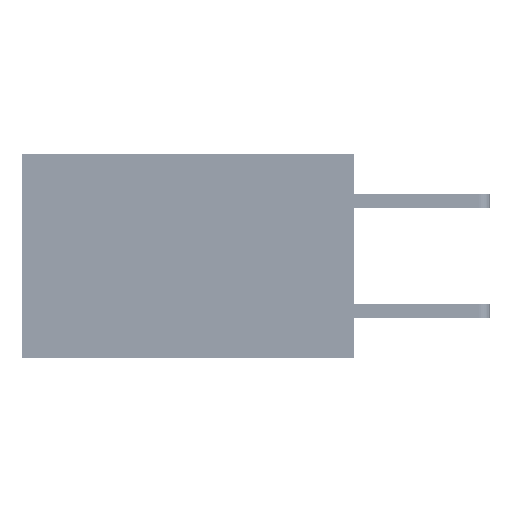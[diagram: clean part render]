
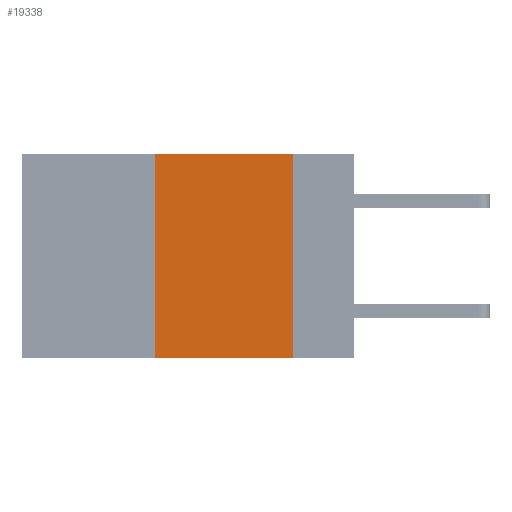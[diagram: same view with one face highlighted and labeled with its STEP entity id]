
A CAD part, left-side view. The second image highlights one B-rep face of the part: STEP entity #19338.
In plain terms, the highlighted planar face has unit normal (-1, 0, 0).
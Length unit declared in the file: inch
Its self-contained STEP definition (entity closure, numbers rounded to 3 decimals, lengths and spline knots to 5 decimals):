
#36 = CARTESIAN_POINT ( 'NONE',  ( 0., 0.11, 0. ) ) ;
#203 = DIRECTION ( 'NONE',  ( 0., -1., 0. ) ) ;
#1530 = VERTEX_POINT ( 'NONE', #18561 ) ;
#1953 = LINE ( 'NONE', #26231, #17473 ) ;
#5167 = ORIENTED_EDGE ( 'NONE', *, *, #29840, .F. ) ;
#6471 = VERTEX_POINT ( 'NONE', #21093 ) ;
#7067 = VECTOR ( 'NONE', #14658, 39.37008 ) ;
#13841 = VECTOR ( 'NONE', #46342, 39.37008 ) ;
#14285 = EDGE_CURVE ( 'NONE', #43423, #21439, #18416, .T. ) ;
#14658 = DIRECTION ( 'NONE',  ( 0., 0., -1. ) ) ;
#16258 = CARTESIAN_POINT ( 'NONE',  ( 0., 0.11, 0. ) ) ;
#16820 = PLANE ( 'NONE',  #38853 ) ;
#17473 = VECTOR ( 'NONE', #40788, 39.37008 ) ;
#18416 = LINE ( 'NONE', #36, #7067 ) ;
#18561 = CARTESIAN_POINT ( 'NONE',  ( 0., 0.36, -0.37 ) ) ;
#19338 = ADVANCED_FACE ( 'NONE', ( #24798 ), #16820, .F. ) ;
#19542 = CARTESIAN_POINT ( 'NONE',  ( 0., 0.11, -0.37 ) ) ;
#20822 = CARTESIAN_POINT ( 'NONE',  ( 0., 0.6, 0. ) ) ;
#21093 = CARTESIAN_POINT ( 'NONE',  ( 0., 0.36, 0. ) ) ;
#21439 = VERTEX_POINT ( 'NONE', #19542 ) ;
#24097 = VECTOR ( 'NONE', #203, 39.37008 ) ;
#24798 = FACE_OUTER_BOUND ( 'NONE', #25071, .T. ) ;
#25071 = EDGE_LOOP ( 'NONE', ( #27466, #32535, #5167, #32768 ) ) ;
#25458 = EDGE_CURVE ( 'NONE', #1530, #21439, #38836, .T. ) ;
#26231 = CARTESIAN_POINT ( 'NONE',  ( 0., 0.6, 0. ) ) ;
#27466 = ORIENTED_EDGE ( 'NONE', *, *, #14285, .F. ) ;
#27683 = EDGE_CURVE ( 'NONE', #6471, #43423, #1953, .T. ) ;
#28952 = CARTESIAN_POINT ( 'NONE',  ( 0., 0.6, -0.37 ) ) ;
#29840 = EDGE_CURVE ( 'NONE', #1530, #6471, #32710, .T. ) ;
#32535 = ORIENTED_EDGE ( 'NONE', *, *, #27683, .F. ) ;
#32710 = LINE ( 'NONE', #43050, #13841 ) ;
#32768 = ORIENTED_EDGE ( 'NONE', *, *, #25458, .T. ) ;
#35156 = DIRECTION ( 'NONE',  ( 1., 0., 0. ) ) ;
#38684 = DIRECTION ( 'NONE',  ( 0., 0., -1. ) ) ;
#38836 = LINE ( 'NONE', #28952, #24097 ) ;
#38853 = AXIS2_PLACEMENT_3D ( 'NONE', #20822, #35156, #38684 ) ;
#40788 = DIRECTION ( 'NONE',  ( 0., -1., 0. ) ) ;
#43050 = CARTESIAN_POINT ( 'NONE',  ( 0., 0.36, 0. ) ) ;
#43423 = VERTEX_POINT ( 'NONE', #16258 ) ;
#46342 = DIRECTION ( 'NONE',  ( 0., 0., 1. ) ) ;
